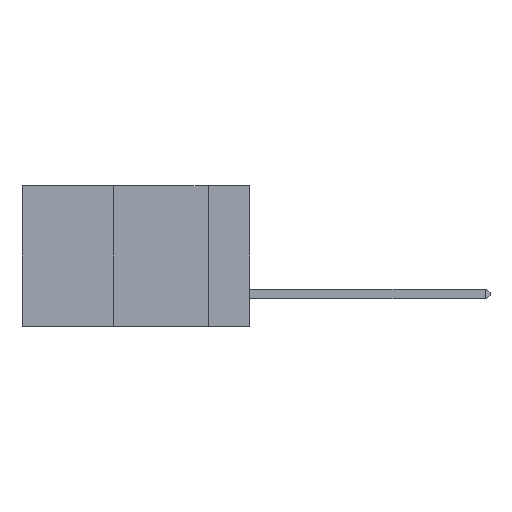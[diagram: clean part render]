
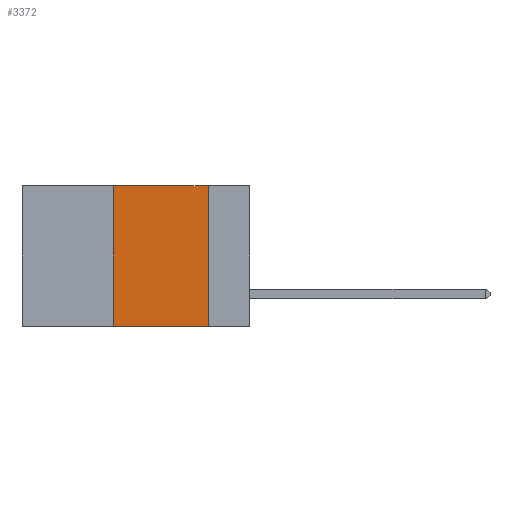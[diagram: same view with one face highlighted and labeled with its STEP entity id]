
A CAD part, left-side view. The second image highlights one B-rep face of the part: STEP entity #3372.
In plain terms, the highlighted planar face has unit normal (-1, 0, 0).
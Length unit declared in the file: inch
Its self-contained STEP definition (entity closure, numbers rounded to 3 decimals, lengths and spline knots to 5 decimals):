
#29 = DIRECTION ( 'NONE',  ( 0., 0., -1. ) ) ;
#86 = CARTESIAN_POINT ( 'NONE',  ( 0., 0.11, -0.37 ) ) ;
#170 = VERTEX_POINT ( 'NONE', #11334 ) ;
#214 = DIRECTION ( 'NONE',  ( 0., 0., -1. ) ) ;
#1238 = DIRECTION ( 'NONE',  ( 0., -1., 0. ) ) ;
#1461 = LINE ( 'NONE', #9801, #6450 ) ;
#1576 = ORIENTED_EDGE ( 'NONE', *, *, #10354, .F. ) ;
#1659 = VECTOR ( 'NONE', #1238, 39.37008 ) ;
#2150 = EDGE_LOOP ( 'NONE', ( #9073, #6937, #1576, #9319 ) ) ;
#2203 = EDGE_CURVE ( 'NONE', #4284, #5564, #5105, .T. ) ;
#2345 = VECTOR ( 'NONE', #2973, 39.37008 ) ;
#2973 = DIRECTION ( 'NONE',  ( 0., 0., 1. ) ) ;
#3372 = ADVANCED_FACE ( 'NONE', ( #6543 ), #10108, .F. ) ;
#3833 = EDGE_CURVE ( 'NONE', #170, #10510, #7024, .T. ) ;
#4284 = VERTEX_POINT ( 'NONE', #5907 ) ;
#5105 = LINE ( 'NONE', #10374, #11308 ) ;
#5564 = VERTEX_POINT ( 'NONE', #5974 ) ;
#5907 = CARTESIAN_POINT ( 'NONE',  ( 0., 0.36, 0. ) ) ;
#5974 = CARTESIAN_POINT ( 'NONE',  ( 0., 0.11, 0. ) ) ;
#6450 = VECTOR ( 'NONE', #214, 39.37008 ) ;
#6543 = FACE_OUTER_BOUND ( 'NONE', #2150, .T. ) ;
#6937 = ORIENTED_EDGE ( 'NONE', *, *, #2203, .F. ) ;
#7024 = LINE ( 'NONE', #7650, #1659 ) ;
#7487 = CARTESIAN_POINT ( 'NONE',  ( 0., 0.6, 0. ) ) ;
#7650 = CARTESIAN_POINT ( 'NONE',  ( 0., 0.6, -0.37 ) ) ;
#7879 = AXIS2_PLACEMENT_3D ( 'NONE', #7487, #8365, #29 ) ;
#8365 = DIRECTION ( 'NONE',  ( 1., 0., 0. ) ) ;
#8803 = CARTESIAN_POINT ( 'NONE',  ( 0., 0.36, 0. ) ) ;
#9010 = EDGE_CURVE ( 'NONE', #5564, #10510, #1461, .T. ) ;
#9073 = ORIENTED_EDGE ( 'NONE', *, *, #9010, .F. ) ;
#9075 = DIRECTION ( 'NONE',  ( 0., -1., 0. ) ) ;
#9319 = ORIENTED_EDGE ( 'NONE', *, *, #3833, .T. ) ;
#9801 = CARTESIAN_POINT ( 'NONE',  ( 0., 0.11, 0. ) ) ;
#10108 = PLANE ( 'NONE',  #7879 ) ;
#10354 = EDGE_CURVE ( 'NONE', #170, #4284, #10891, .T. ) ;
#10374 = CARTESIAN_POINT ( 'NONE',  ( 0., 0.6, 0. ) ) ;
#10510 = VERTEX_POINT ( 'NONE', #86 ) ;
#10891 = LINE ( 'NONE', #8803, #2345 ) ;
#11308 = VECTOR ( 'NONE', #9075, 39.37008 ) ;
#11334 = CARTESIAN_POINT ( 'NONE',  ( 0., 0.36, -0.37 ) ) ;
